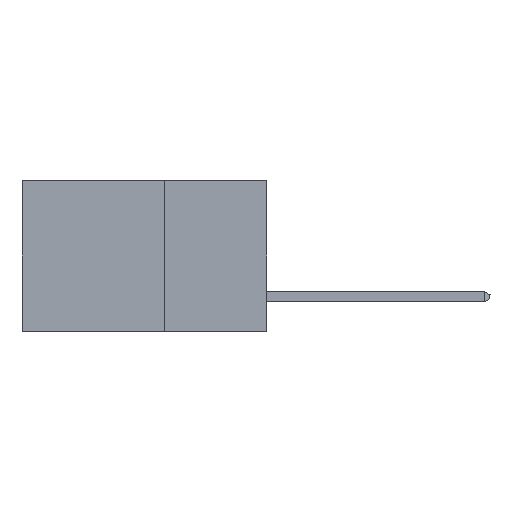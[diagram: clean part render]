
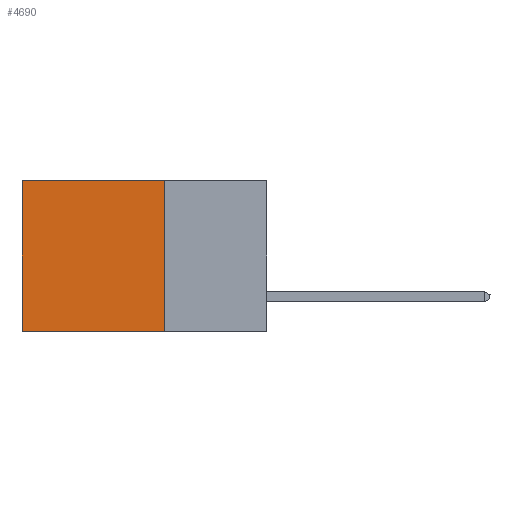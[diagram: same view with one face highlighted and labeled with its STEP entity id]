
A CAD part, left-side view. The second image highlights one B-rep face of the part: STEP entity #4690.
In plain terms, the highlighted planar face has unit normal (-1, 0, 0).
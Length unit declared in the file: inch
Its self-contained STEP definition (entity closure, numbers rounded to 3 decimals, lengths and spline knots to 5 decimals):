
#1941 = ORIENTED_EDGE ( 'NONE', *, *, #24555, .T. ) ;
#3455 = LINE ( 'NONE', #13420, #33550 ) ;
#4690 = ADVANCED_FACE ( 'NONE', ( #21406 ), #21628, .F. ) ;
#4917 = VERTEX_POINT ( 'NONE', #24352 ) ;
#5849 = CARTESIAN_POINT ( 'NONE',  ( 0.2875, 0.6, 0. ) ) ;
#7519 = DIRECTION ( 'NONE',  ( 1., 0., 0. ) ) ;
#7533 = EDGE_CURVE ( 'NONE', #34796, #4917, #16821, .T. ) ;
#7959 = CARTESIAN_POINT ( 'NONE',  ( 0.2875, 0.6, -0.37 ) ) ;
#8332 = AXIS2_PLACEMENT_3D ( 'NONE', #15152, #7519, #39630 ) ;
#9308 = LINE ( 'NONE', #5849, #23505 ) ;
#9595 = CARTESIAN_POINT ( 'NONE',  ( 0.2875, 0.25, -0.37 ) ) ;
#10211 = EDGE_CURVE ( 'NONE', #34796, #30094, #3455, .T. ) ;
#10366 = ORIENTED_EDGE ( 'NONE', *, *, #7533, .T. ) ;
#10631 = EDGE_CURVE ( 'NONE', #30094, #24381, #23471, .T. ) ;
#11521 = EDGE_LOOP ( 'NONE', ( #1941, #42558, #28471, #10366 ) ) ;
#13420 = CARTESIAN_POINT ( 'NONE',  ( 0.2875, 0.25, 0. ) ) ;
#14838 = CARTESIAN_POINT ( 'NONE',  ( 0.2875, 0.25, -0.37 ) ) ;
#15152 = CARTESIAN_POINT ( 'NONE',  ( 0.2875, 0.25, 0. ) ) ;
#16254 = DIRECTION ( 'NONE',  ( 0., 0., -1. ) ) ;
#16821 = LINE ( 'NONE', #30670, #20330 ) ;
#17582 = DIRECTION ( 'NONE',  ( 0., 0., -1. ) ) ;
#20330 = VECTOR ( 'NONE', #23981, 39.37008 ) ;
#21406 = FACE_OUTER_BOUND ( 'NONE', #11521, .T. ) ;
#21628 = PLANE ( 'NONE',  #8332 ) ;
#23471 = LINE ( 'NONE', #9595, #42423 ) ;
#23505 = VECTOR ( 'NONE', #16254, 39.37008 ) ;
#23981 = DIRECTION ( 'NONE',  ( 0., 1., 0. ) ) ;
#24352 = CARTESIAN_POINT ( 'NONE',  ( 0.2875, 0.6, 0. ) ) ;
#24370 = DIRECTION ( 'NONE',  ( 0., 1., 0. ) ) ;
#24381 = VERTEX_POINT ( 'NONE', #7959 ) ;
#24555 = EDGE_CURVE ( 'NONE', #4917, #24381, #9308, .T. ) ;
#28471 = ORIENTED_EDGE ( 'NONE', *, *, #10211, .F. ) ;
#30094 = VERTEX_POINT ( 'NONE', #14838 ) ;
#30670 = CARTESIAN_POINT ( 'NONE',  ( 0.2875, 0.25, 0. ) ) ;
#33550 = VECTOR ( 'NONE', #17582, 39.37008 ) ;
#34778 = CARTESIAN_POINT ( 'NONE',  ( 0.2875, 0.25, 0. ) ) ;
#34796 = VERTEX_POINT ( 'NONE', #34778 ) ;
#39630 = DIRECTION ( 'NONE',  ( 0., 0., -1. ) ) ;
#42423 = VECTOR ( 'NONE', #24370, 39.37008 ) ;
#42558 = ORIENTED_EDGE ( 'NONE', *, *, #10631, .F. ) ;
